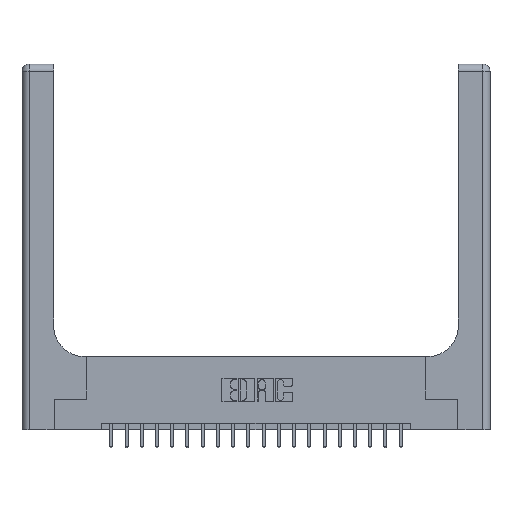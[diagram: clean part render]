
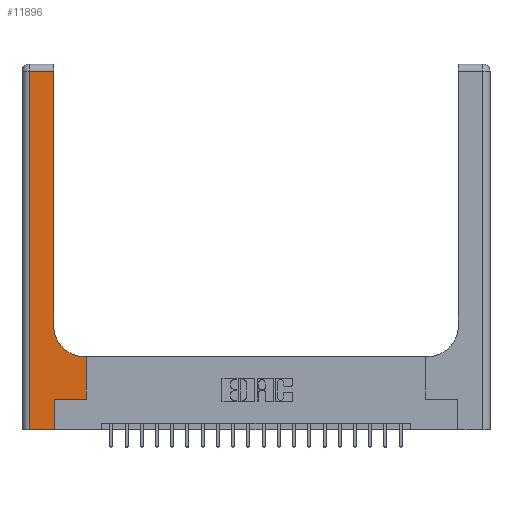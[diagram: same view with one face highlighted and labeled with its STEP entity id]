
A CAD part, top view. The second image highlights one B-rep face of the part: STEP entity #11896.
In plain terms, the highlighted planar face has unit normal (0, 0, 1).
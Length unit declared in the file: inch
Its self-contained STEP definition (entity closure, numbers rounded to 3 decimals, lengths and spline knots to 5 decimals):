
#420 = VERTEX_POINT ( 'NONE', #12740 ) ;
#432 = CARTESIAN_POINT ( 'NONE',  ( 0.06, 3., 0.37 ) ) ;
#661 = DIRECTION ( 'NONE',  ( -1., 0., 0. ) ) ;
#719 = CARTESIAN_POINT ( 'NONE',  ( 0.528, 0.25, 0.37 ) ) ;
#1210 = VECTOR ( 'NONE', #1360, 39.37008 ) ;
#1360 = DIRECTION ( 'NONE',  ( -1., 0., 0. ) ) ;
#1674 = DIRECTION ( 'NONE',  ( 0., 1., 0. ) ) ;
#2314 = EDGE_CURVE ( 'NONE', #12821, #420, #5342, .T. ) ;
#2344 = LINE ( 'NONE', #5210, #16950 ) ;
#2557 = CIRCLE ( 'NONE', #16554, 0.25 ) ;
#2763 = FACE_OUTER_BOUND ( 'NONE', #14723, .T. ) ;
#2894 = VERTEX_POINT ( 'NONE', #4733 ) ;
#4733 = CARTESIAN_POINT ( 'NONE',  ( 0.06, 2.94, 0.37 ) ) ;
#4753 = VECTOR ( 'NONE', #1674, 39.37008 ) ;
#5210 = CARTESIAN_POINT ( 'NONE',  ( 0.265, 0.25, 0.37 ) ) ;
#5342 = LINE ( 'NONE', #6992, #8096 ) ;
#5499 = AXIS2_PLACEMENT_3D ( 'NONE', #7797, #14122, #661 ) ;
#6397 = LINE ( 'NONE', #16670, #4753 ) ;
#6519 = ORIENTED_EDGE ( 'NONE', *, *, #14952, .T. ) ;
#6672 = ORIENTED_EDGE ( 'NONE', *, *, #9283, .T. ) ;
#6673 = DIRECTION ( 'NONE',  ( 1., 0., 0. ) ) ;
#6992 = CARTESIAN_POINT ( 'NONE',  ( 0., 0., 0.37 ) ) ;
#7402 = DIRECTION ( 'NONE',  ( 0., 1., 0. ) ) ;
#7690 = CARTESIAN_POINT ( 'NONE',  ( 0.265, 0.25, 0.37 ) ) ;
#7797 = CARTESIAN_POINT ( 'NONE',  ( 0., 3., 0.37 ) ) ;
#8096 = VECTOR ( 'NONE', #6673, 39.37008 ) ;
#8170 = LINE ( 'NONE', #14822, #9334 ) ;
#8279 = VERTEX_POINT ( 'NONE', #20882 ) ;
#8354 = VERTEX_POINT ( 'NONE', #13096 ) ;
#8516 = EDGE_CURVE ( 'NONE', #16278, #14978, #2344, .T. ) ;
#8658 = ORIENTED_EDGE ( 'NONE', *, *, #2314, .T. ) ;
#8702 = DIRECTION ( 'NONE',  ( 1., 0., 0. ) ) ;
#9283 = EDGE_CURVE ( 'NONE', #2894, #12821, #15426, .T. ) ;
#9316 = PLANE ( 'NONE',  #5499 ) ;
#9334 = VECTOR ( 'NONE', #10016, 39.37008 ) ;
#10016 = DIRECTION ( 'NONE',  ( 0., 1., 0. ) ) ;
#10331 = EDGE_CURVE ( 'NONE', #18901, #11260, #12848, .T. ) ;
#10470 = ORIENTED_EDGE ( 'NONE', *, *, #10957, .T. ) ;
#10957 = EDGE_CURVE ( 'NONE', #14978, #18901, #20339, .T. ) ;
#11134 = ORIENTED_EDGE ( 'NONE', *, *, #20619, .T. ) ;
#11260 = VERTEX_POINT ( 'NONE', #13414 ) ;
#11896 = ADVANCED_FACE ( 'NONE', ( #2763 ), #9316, .F. ) ;
#11931 = ORIENTED_EDGE ( 'NONE', *, *, #10331, .T. ) ;
#11987 = CARTESIAN_POINT ( 'NONE',  ( 0.528, 0.25, 0.37 ) ) ;
#12361 = VECTOR ( 'NONE', #20632, 39.37008 ) ;
#12740 = CARTESIAN_POINT ( 'NONE',  ( 0.265, 0., 0.37 ) ) ;
#12821 = VERTEX_POINT ( 'NONE', #19418 ) ;
#12848 = LINE ( 'NONE', #14805, #1210 ) ;
#13096 = CARTESIAN_POINT ( 'NONE',  ( 0.26, 2.94, 0.37 ) ) ;
#13394 = EDGE_CURVE ( 'NONE', #420, #16278, #6397, .T. ) ;
#13414 = CARTESIAN_POINT ( 'NONE',  ( 0.51, 0.6, 0.37 ) ) ;
#13522 = LINE ( 'NONE', #13728, #12361 ) ;
#13564 = VECTOR ( 'NONE', #18405, 39.37008 ) ;
#13728 = CARTESIAN_POINT ( 'NONE',  ( 0., 2.94, 0.37 ) ) ;
#14122 = DIRECTION ( 'NONE',  ( 0., 0., -1. ) ) ;
#14383 = EDGE_CURVE ( 'NONE', #11260, #8279, #2557, .T. ) ;
#14578 = ORIENTED_EDGE ( 'NONE', *, *, #14383, .T. ) ;
#14723 = EDGE_LOOP ( 'NONE', ( #11134, #6519, #6672, #8658, #14818, #20110, #10470, #11931, #14578 ) ) ;
#14805 = CARTESIAN_POINT ( 'NONE',  ( 0.26, 0.6, 0.37 ) ) ;
#14818 = ORIENTED_EDGE ( 'NONE', *, *, #13394, .T. ) ;
#14822 = CARTESIAN_POINT ( 'NONE',  ( 0.26, 3., 0.37 ) ) ;
#14952 = EDGE_CURVE ( 'NONE', #8354, #2894, #13522, .T. ) ;
#14978 = VERTEX_POINT ( 'NONE', #11987 ) ;
#15426 = LINE ( 'NONE', #432, #13564 ) ;
#15840 = VECTOR ( 'NONE', #7402, 39.37008 ) ;
#16220 = DIRECTION ( 'NONE',  ( 1., 0., 0. ) ) ;
#16278 = VERTEX_POINT ( 'NONE', #7690 ) ;
#16423 = CARTESIAN_POINT ( 'NONE',  ( 0.528, 0.6, 0.37 ) ) ;
#16554 = AXIS2_PLACEMENT_3D ( 'NONE', #19493, #21377, #16220 ) ;
#16670 = CARTESIAN_POINT ( 'NONE',  ( 0.265, 0., 0.37 ) ) ;
#16950 = VECTOR ( 'NONE', #8702, 39.37008 ) ;
#18405 = DIRECTION ( 'NONE',  ( 0., -1., 0. ) ) ;
#18901 = VERTEX_POINT ( 'NONE', #16423 ) ;
#19418 = CARTESIAN_POINT ( 'NONE',  ( 0.06, 0., 0.37 ) ) ;
#19493 = CARTESIAN_POINT ( 'NONE',  ( 0.51, 0.85, 0.37 ) ) ;
#20110 = ORIENTED_EDGE ( 'NONE', *, *, #8516, .T. ) ;
#20339 = LINE ( 'NONE', #719, #15840 ) ;
#20619 = EDGE_CURVE ( 'NONE', #8279, #8354, #8170, .T. ) ;
#20632 = DIRECTION ( 'NONE',  ( -1., 0., 0. ) ) ;
#20882 = CARTESIAN_POINT ( 'NONE',  ( 0.26, 0.85, 0.37 ) ) ;
#21377 = DIRECTION ( 'NONE',  ( 0., 0., -1. ) ) ;
